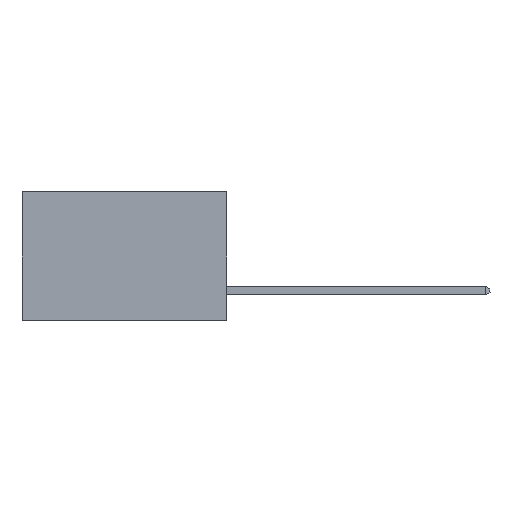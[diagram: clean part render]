
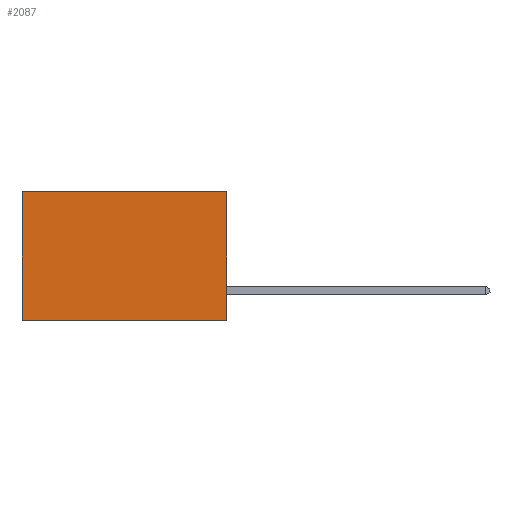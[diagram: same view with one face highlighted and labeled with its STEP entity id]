
A CAD part, left-side view. The second image highlights one B-rep face of the part: STEP entity #2087.
In plain terms, the highlighted planar face has unit normal (-1, 0, 0).
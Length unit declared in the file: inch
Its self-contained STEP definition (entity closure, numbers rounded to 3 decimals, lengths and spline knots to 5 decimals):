
#139 = VECTOR ( 'NONE', #7240, 39.37008 ) ;
#392 = DIRECTION ( 'NONE',  ( 1., 0., 0. ) ) ;
#871 = ORIENTED_EDGE ( 'NONE', *, *, #6537, .T. ) ;
#919 = CARTESIAN_POINT ( 'NONE',  ( 0.277, 0.59, 0. ) ) ;
#1072 = VERTEX_POINT ( 'NONE', #12187 ) ;
#1748 = CARTESIAN_POINT ( 'NONE',  ( 0.277, 0., -0.37 ) ) ;
#1855 = CARTESIAN_POINT ( 'NONE',  ( 0.277, 0.59, -0.37 ) ) ;
#2087 = ADVANCED_FACE ( 'NONE', ( #9194 ), #5949, .F. ) ;
#2165 = CARTESIAN_POINT ( 'NONE',  ( 0.277, 0., 0. ) ) ;
#2327 = DIRECTION ( 'NONE',  ( 0., 1., 0. ) ) ;
#3063 = EDGE_CURVE ( 'NONE', #7303, #9865, #7548, .T. ) ;
#3404 = LINE ( 'NONE', #8167, #139 ) ;
#3509 = VECTOR ( 'NONE', #13623, 39.37008 ) ;
#3729 = EDGE_LOOP ( 'NONE', ( #871, #5237, #6739, #5070 ) ) ;
#3795 = EDGE_CURVE ( 'NONE', #1072, #7303, #3404, .T. ) ;
#4312 = EDGE_CURVE ( 'NONE', #1072, #5430, #14669, .T. ) ;
#4771 = AXIS2_PLACEMENT_3D ( 'NONE', #7477, #392, #9332 ) ;
#5070 = ORIENTED_EDGE ( 'NONE', *, *, #4312, .T. ) ;
#5237 = ORIENTED_EDGE ( 'NONE', *, *, #3063, .F. ) ;
#5289 = DIRECTION ( 'NONE',  ( 0., 1., 0. ) ) ;
#5430 = VERTEX_POINT ( 'NONE', #919 ) ;
#5949 = PLANE ( 'NONE',  #4771 ) ;
#6537 = EDGE_CURVE ( 'NONE', #5430, #9865, #7048, .T. ) ;
#6739 = ORIENTED_EDGE ( 'NONE', *, *, #3795, .F. ) ;
#6826 = CARTESIAN_POINT ( 'NONE',  ( 0.277, 0., -0.37 ) ) ;
#7048 = LINE ( 'NONE', #13555, #3509 ) ;
#7240 = DIRECTION ( 'NONE',  ( 0., 0., -1. ) ) ;
#7303 = VERTEX_POINT ( 'NONE', #6826 ) ;
#7477 = CARTESIAN_POINT ( 'NONE',  ( 0.277, 0., -0.37 ) ) ;
#7548 = LINE ( 'NONE', #1748, #13190 ) ;
#7855 = VECTOR ( 'NONE', #2327, 39.37008 ) ;
#8167 = CARTESIAN_POINT ( 'NONE',  ( 0.277, 0., -0.37 ) ) ;
#9194 = FACE_OUTER_BOUND ( 'NONE', #3729, .T. ) ;
#9332 = DIRECTION ( 'NONE',  ( 0., 0., -1. ) ) ;
#9865 = VERTEX_POINT ( 'NONE', #1855 ) ;
#12187 = CARTESIAN_POINT ( 'NONE',  ( 0.277, 0., 0. ) ) ;
#13190 = VECTOR ( 'NONE', #5289, 39.37008 ) ;
#13555 = CARTESIAN_POINT ( 'NONE',  ( 0.277, 0.59, -0.37 ) ) ;
#13623 = DIRECTION ( 'NONE',  ( 0., 0., -1. ) ) ;
#14669 = LINE ( 'NONE', #2165, #7855 ) ;
